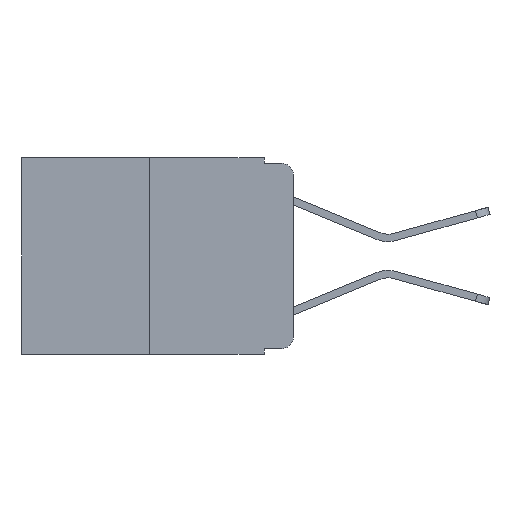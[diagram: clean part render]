
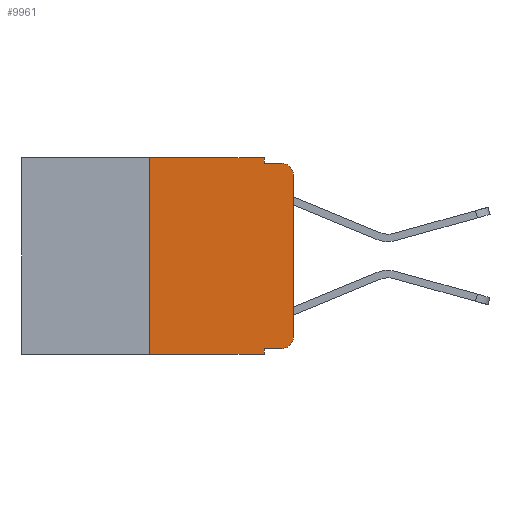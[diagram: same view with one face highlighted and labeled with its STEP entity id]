
A CAD part, left-side view. The second image highlights one B-rep face of the part: STEP entity #9961.
In plain terms, the highlighted planar face has unit normal (-1, 0, 0).
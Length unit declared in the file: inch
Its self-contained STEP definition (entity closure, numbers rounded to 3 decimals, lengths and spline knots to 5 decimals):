
#406 = CARTESIAN_POINT ( 'NONE',  ( 0., 0.473, 0. ) ) ;
#1327 = CARTESIAN_POINT ( 'NONE',  ( 0., 0.473, 0. ) ) ;
#1465 = VERTEX_POINT ( 'NONE', #15500 ) ;
#1591 = CARTESIAN_POINT ( 'NONE',  ( 0., 0.051, -0.333 ) ) ;
#1708 = ORIENTED_EDGE ( 'NONE', *, *, #16946, .F. ) ;
#1797 = CARTESIAN_POINT ( 'NONE',  ( 0., 0.051, -0.01 ) ) ;
#1860 = CARTESIAN_POINT ( 'NONE',  ( 0., 0.25, 0. ) ) ;
#1889 = FACE_OUTER_BOUND ( 'NONE', #3505, .T. ) ;
#1953 = VECTOR ( 'NONE', #3170, 39.37008 ) ;
#2217 = EDGE_CURVE ( 'NONE', #21178, #18951, #19648, .T. ) ;
#2305 = DIRECTION ( 'NONE',  ( 1., 0., 0. ) ) ;
#2406 = LINE ( 'NONE', #20263, #7632 ) ;
#2461 = LINE ( 'NONE', #16365, #10615 ) ;
#2730 = ORIENTED_EDGE ( 'NONE', *, *, #17481, .F. ) ;
#2857 = CARTESIAN_POINT ( 'NONE',  ( 0., 0.051, 0. ) ) ;
#2960 = AXIS2_PLACEMENT_3D ( 'NONE', #7322, #18998, #9046 ) ;
#3170 = DIRECTION ( 'NONE',  ( 0., -1., 0. ) ) ;
#3275 = VECTOR ( 'NONE', #15579, 39.37008 ) ;
#3305 = CARTESIAN_POINT ( 'NONE',  ( 0., 0.25, 0. ) ) ;
#3413 = EDGE_CURVE ( 'NONE', #4212, #21178, #16652, .T. ) ;
#3505 = EDGE_LOOP ( 'NONE', ( #21693, #17448, #9657, #15645, #1708, #15428, #11103, #2730, #17608, #3565 ) ) ;
#3565 = ORIENTED_EDGE ( 'NONE', *, *, #15262, .T. ) ;
#4212 = VERTEX_POINT ( 'NONE', #17924 ) ;
#4466 = VERTEX_POINT ( 'NONE', #3305 ) ;
#4612 = DIRECTION ( 'NONE',  ( 0., 0., -1. ) ) ;
#5581 = CARTESIAN_POINT ( 'NONE',  ( 0., 0., 0. ) ) ;
#6316 = CARTESIAN_POINT ( 'NONE',  ( 0., 0.051, -0.01 ) ) ;
#6571 = VERTEX_POINT ( 'NONE', #1797 ) ;
#7012 = DIRECTION ( 'NONE',  ( 0., -1., 0. ) ) ;
#7322 = CARTESIAN_POINT ( 'NONE',  ( 0., 0.02, -0.03 ) ) ;
#7544 = PLANE ( 'NONE',  #17659 ) ;
#7632 = VECTOR ( 'NONE', #7012, 39.37008 ) ;
#7940 = LINE ( 'NONE', #1860, #3275 ) ;
#8028 = DIRECTION ( 'NONE',  ( 0., 0., -1. ) ) ;
#8157 = VECTOR ( 'NONE', #11463, 39.37008 ) ;
#8958 = AXIS2_PLACEMENT_3D ( 'NONE', #10523, #22111, #12201 ) ;
#9046 = DIRECTION ( 'NONE',  ( 0., 0., -1. ) ) ;
#9657 = ORIENTED_EDGE ( 'NONE', *, *, #21918, .F. ) ;
#9930 = LINE ( 'NONE', #1591, #17722 ) ;
#9961 = ADVANCED_FACE ( 'NONE', ( #1889 ), #7544, .F. ) ;
#10523 = CARTESIAN_POINT ( 'NONE',  ( 0., 0.02, -0.313 ) ) ;
#10615 = VECTOR ( 'NONE', #8028, 39.37008 ) ;
#10998 = VERTEX_POINT ( 'NONE', #21263 ) ;
#11103 = ORIENTED_EDGE ( 'NONE', *, *, #13336, .T. ) ;
#11140 = CARTESIAN_POINT ( 'NONE',  ( 0., 0., -0.03 ) ) ;
#11223 = LINE ( 'NONE', #1327, #1953 ) ;
#11449 = VERTEX_POINT ( 'NONE', #21160 ) ;
#11463 = DIRECTION ( 'NONE',  ( 0., -1., 0. ) ) ;
#12201 = DIRECTION ( 'NONE',  ( 0., 0., -1. ) ) ;
#13024 = VECTOR ( 'NONE', #4612, 39.37008 ) ;
#13336 = EDGE_CURVE ( 'NONE', #1465, #10998, #2406, .T. ) ;
#13627 = CARTESIAN_POINT ( 'NONE',  ( 0., 0.051, 0. ) ) ;
#14317 = DIRECTION ( 'NONE',  ( 0., 0., -1. ) ) ;
#15186 = CIRCLE ( 'NONE', #8958, 0.02 ) ;
#15262 = EDGE_CURVE ( 'NONE', #11449, #4212, #15186, .T. ) ;
#15342 = DIRECTION ( 'NONE',  ( 0., -1., 0. ) ) ;
#15428 = ORIENTED_EDGE ( 'NONE', *, *, #18575, .F. ) ;
#15500 = CARTESIAN_POINT ( 'NONE',  ( 0., 0.25, -0.343 ) ) ;
#15579 = DIRECTION ( 'NONE',  ( 0., 0., 1. ) ) ;
#15645 = ORIENTED_EDGE ( 'NONE', *, *, #20748, .F. ) ;
#16080 = CARTESIAN_POINT ( 'NONE',  ( 0., 0.051, -0.333 ) ) ;
#16365 = CARTESIAN_POINT ( 'NONE',  ( 0., 0.051, 0. ) ) ;
#16380 = EDGE_CURVE ( 'NONE', #18760, #11449, #9930, .T. ) ;
#16580 = CARTESIAN_POINT ( 'NONE',  ( 0., 0.02, -0.01 ) ) ;
#16652 = LINE ( 'NONE', #5581, #19489 ) ;
#16946 = EDGE_CURVE ( 'NONE', #4466, #20360, #11223, .T. ) ;
#17448 = ORIENTED_EDGE ( 'NONE', *, *, #2217, .T. ) ;
#17481 = EDGE_CURVE ( 'NONE', #18760, #10998, #21815, .T. ) ;
#17608 = ORIENTED_EDGE ( 'NONE', *, *, #16380, .T. ) ;
#17659 = AXIS2_PLACEMENT_3D ( 'NONE', #406, #2305, #14317 ) ;
#17722 = VECTOR ( 'NONE', #15342, 39.37008 ) ;
#17924 = CARTESIAN_POINT ( 'NONE',  ( 0., 0., -0.313 ) ) ;
#18575 = EDGE_CURVE ( 'NONE', #1465, #4466, #7940, .T. ) ;
#18760 = VERTEX_POINT ( 'NONE', #16080 ) ;
#18951 = VERTEX_POINT ( 'NONE', #16580 ) ;
#18998 = DIRECTION ( 'NONE',  ( -1., 0., 0. ) ) ;
#19019 = DIRECTION ( 'NONE',  ( 0., 0., 1. ) ) ;
#19489 = VECTOR ( 'NONE', #19019, 39.37008 ) ;
#19648 = CIRCLE ( 'NONE', #2960, 0.02 ) ;
#20263 = CARTESIAN_POINT ( 'NONE',  ( 0., 0.473, -0.343 ) ) ;
#20360 = VERTEX_POINT ( 'NONE', #13627 ) ;
#20748 = EDGE_CURVE ( 'NONE', #20360, #6571, #2461, .T. ) ;
#21160 = CARTESIAN_POINT ( 'NONE',  ( 0., 0.02, -0.333 ) ) ;
#21178 = VERTEX_POINT ( 'NONE', #11140 ) ;
#21263 = CARTESIAN_POINT ( 'NONE',  ( 0., 0.051, -0.343 ) ) ;
#21431 = LINE ( 'NONE', #6316, #8157 ) ;
#21693 = ORIENTED_EDGE ( 'NONE', *, *, #3413, .T. ) ;
#21815 = LINE ( 'NONE', #2857, #13024 ) ;
#21918 = EDGE_CURVE ( 'NONE', #6571, #18951, #21431, .T. ) ;
#22111 = DIRECTION ( 'NONE',  ( -1., 0., 0. ) ) ;
